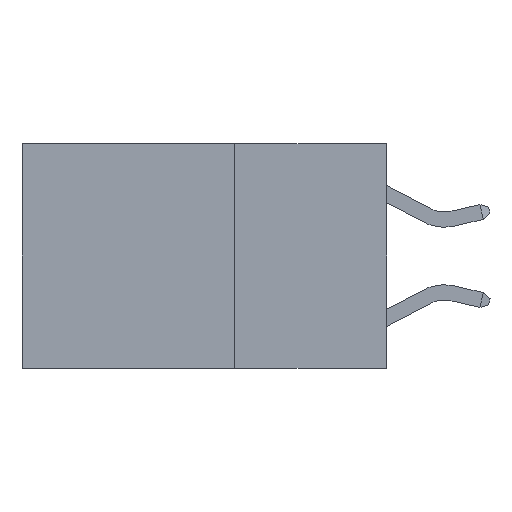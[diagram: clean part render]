
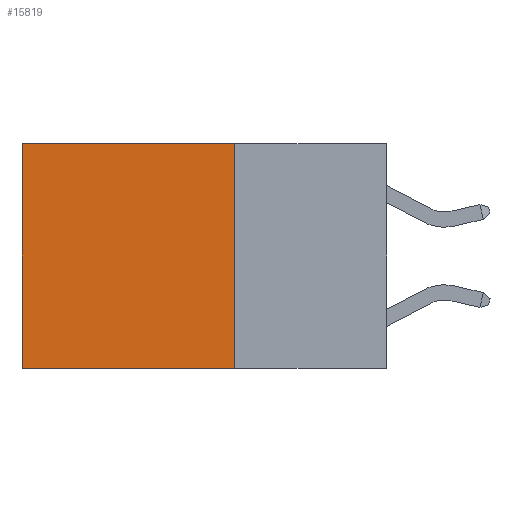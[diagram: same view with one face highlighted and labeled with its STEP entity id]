
A CAD part, left-side view. The second image highlights one B-rep face of the part: STEP entity #15819.
In plain terms, the highlighted planar face has unit normal (-1, 0, 0).
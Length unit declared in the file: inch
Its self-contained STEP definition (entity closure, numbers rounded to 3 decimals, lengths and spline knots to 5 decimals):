
#326 = DIRECTION ( 'NONE',  ( 0., 0., -1. ) ) ;
#500 = PLANE ( 'NONE',  #11630 ) ;
#667 = VECTOR ( 'NONE', #9801, 39.37008 ) ;
#1084 = EDGE_CURVE ( 'NONE', #17315, #2703, #2017, .T. ) ;
#2017 = LINE ( 'NONE', #15451, #14626 ) ;
#2062 = FACE_OUTER_BOUND ( 'NONE', #19025, .T. ) ;
#2204 = EDGE_CURVE ( 'NONE', #17315, #7661, #15746, .T. ) ;
#2703 = VERTEX_POINT ( 'NONE', #3467 ) ;
#3467 = CARTESIAN_POINT ( 'NONE',  ( 0.2625, 0.25, -0.37 ) ) ;
#3710 = EDGE_CURVE ( 'NONE', #2703, #25476, #31655, .T. ) ;
#3979 = CARTESIAN_POINT ( 'NONE',  ( 0.2625, 0.25, 0. ) ) ;
#4165 = DIRECTION ( 'NONE',  ( 0., 1., 0. ) ) ;
#5320 = ORIENTED_EDGE ( 'NONE', *, *, #1084, .F. ) ;
#5595 = DIRECTION ( 'NONE',  ( 1., 0., 0. ) ) ;
#7661 = VERTEX_POINT ( 'NONE', #21905 ) ;
#9801 = DIRECTION ( 'NONE',  ( 0., 1., 0. ) ) ;
#10102 = VECTOR ( 'NONE', #17215, 39.37008 ) ;
#11505 = ORIENTED_EDGE ( 'NONE', *, *, #3710, .F. ) ;
#11630 = AXIS2_PLACEMENT_3D ( 'NONE', #20528, #5595, #23187 ) ;
#14626 = VECTOR ( 'NONE', #326, 39.37008 ) ;
#15451 = CARTESIAN_POINT ( 'NONE',  ( 0.2625, 0.25, 0. ) ) ;
#15746 = LINE ( 'NONE', #19204, #28276 ) ;
#15819 = ADVANCED_FACE ( 'NONE', ( #2062 ), #500, .F. ) ;
#17215 = DIRECTION ( 'NONE',  ( 0., 0., -1. ) ) ;
#17315 = VERTEX_POINT ( 'NONE', #3979 ) ;
#19025 = EDGE_LOOP ( 'NONE', ( #32260, #11505, #5320, #22620 ) ) ;
#19204 = CARTESIAN_POINT ( 'NONE',  ( 0.2625, 0.25, 0. ) ) ;
#20174 = EDGE_CURVE ( 'NONE', #7661, #25476, #23465, .T. ) ;
#20528 = CARTESIAN_POINT ( 'NONE',  ( 0.2625, 0.25, 0. ) ) ;
#21905 = CARTESIAN_POINT ( 'NONE',  ( 0.2625, 0.6, 0. ) ) ;
#22261 = CARTESIAN_POINT ( 'NONE',  ( 0.2625, 0.6, 0. ) ) ;
#22592 = CARTESIAN_POINT ( 'NONE',  ( 0.2625, 0.6, -0.37 ) ) ;
#22620 = ORIENTED_EDGE ( 'NONE', *, *, #2204, .T. ) ;
#23187 = DIRECTION ( 'NONE',  ( 0., 0., -1. ) ) ;
#23465 = LINE ( 'NONE', #22261, #10102 ) ;
#24867 = CARTESIAN_POINT ( 'NONE',  ( 0.2625, 0.25, -0.37 ) ) ;
#25476 = VERTEX_POINT ( 'NONE', #22592 ) ;
#28276 = VECTOR ( 'NONE', #4165, 39.37008 ) ;
#31655 = LINE ( 'NONE', #24867, #667 ) ;
#32260 = ORIENTED_EDGE ( 'NONE', *, *, #20174, .T. ) ;
